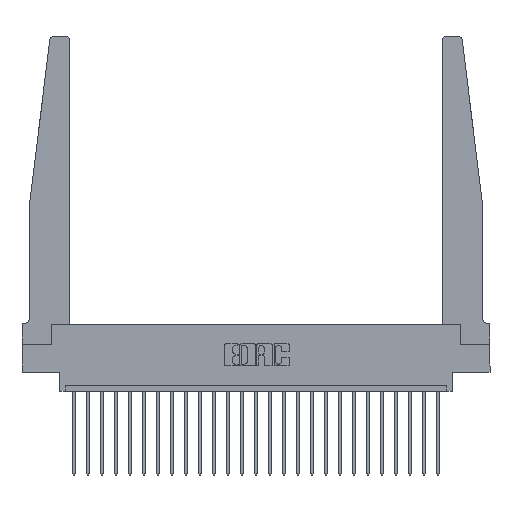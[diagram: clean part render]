
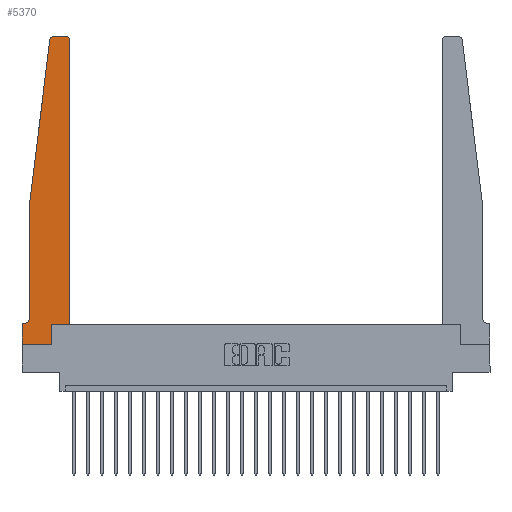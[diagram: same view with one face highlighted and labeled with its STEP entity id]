
A CAD part, top view. The second image highlights one B-rep face of the part: STEP entity #5370.
In plain terms, the highlighted planar face has unit normal (0, 0, 1).
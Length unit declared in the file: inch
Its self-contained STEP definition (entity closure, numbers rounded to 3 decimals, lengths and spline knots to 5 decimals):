
#117 = EDGE_CURVE ( 'NONE', #17860, #14501, #14107, .T. ) ;
#538 = AXIS2_PLACEMENT_3D ( 'NONE', #19461, #14098, #1258 ) ;
#866 = CARTESIAN_POINT ( 'NONE',  ( 0.2605, 0., 0.37 ) ) ;
#1106 = VECTOR ( 'NONE', #4166, 39.37008 ) ;
#1123 = AXIS2_PLACEMENT_3D ( 'NONE', #10240, #10121, #8539 ) ;
#1258 = DIRECTION ( 'NONE',  ( 1., 0., 0. ) ) ;
#1379 = LINE ( 'NONE', #3693, #8368 ) ;
#1719 = CARTESIAN_POINT ( 'NONE',  ( 0., 0., 0.37 ) ) ;
#1880 = DIRECTION ( 'NONE',  ( 0., -1., 0. ) ) ;
#2610 = AXIS2_PLACEMENT_3D ( 'NONE', #13064, #20389, #16616 ) ;
#2617 = DIRECTION ( 'NONE',  ( 0., 1., 0. ) ) ;
#2806 = ORIENTED_EDGE ( 'NONE', *, *, #21294, .T. ) ;
#2955 = VECTOR ( 'NONE', #18451, 39.37008 ) ;
#3635 = VERTEX_POINT ( 'NONE', #22737 ) ;
#3693 = CARTESIAN_POINT ( 'NONE',  ( 0.065, 1.25, 0.37 ) ) ;
#3705 = ORIENTED_EDGE ( 'NONE', *, *, #21782, .T. ) ;
#4132 = CARTESIAN_POINT ( 'NONE',  ( 0., 0., 0.37 ) ) ;
#4146 = ORIENTED_EDGE ( 'NONE', *, *, #23556, .T. ) ;
#4166 = DIRECTION ( 'NONE',  ( 0., 1., 0. ) ) ;
#4489 = ORIENTED_EDGE ( 'NONE', *, *, #9427, .T. ) ;
#4519 = EDGE_CURVE ( 'NONE', #5183, #11745, #11567, .T. ) ;
#4867 = VECTOR ( 'NONE', #2617, 39.37008 ) ;
#4907 = CARTESIAN_POINT ( 'NONE',  ( 0.065, 1.25, 0.37 ) ) ;
#4926 = VECTOR ( 'NONE', #9857, 39.37008 ) ;
#4960 = LINE ( 'NONE', #6920, #7744 ) ;
#5116 = CARTESIAN_POINT ( 'NONE',  ( 0.065, 0.2375, 0.37 ) ) ;
#5183 = VERTEX_POINT ( 'NONE', #22739 ) ;
#5370 = ADVANCED_FACE ( 'NONE', ( #12104 ), #11985, .T. ) ;
#5738 = EDGE_CURVE ( 'NONE', #11604, #5183, #4960, .T. ) ;
#5764 = VECTOR ( 'NONE', #16285, 39.37008 ) ;
#6403 = CARTESIAN_POINT ( 'NONE',  ( 0.425, 0.18, 0.37 ) ) ;
#6478 = DIRECTION ( 'NONE',  ( 1., 0., 0. ) ) ;
#6920 = CARTESIAN_POINT ( 'NONE',  ( 0.065, 0.1875, 0.37 ) ) ;
#7546 = DIRECTION ( 'NONE',  ( 0., -1., 0. ) ) ;
#7744 = VECTOR ( 'NONE', #14486, 39.37008 ) ;
#7966 = CIRCLE ( 'NONE', #538, 0.03 ) ;
#8003 = LINE ( 'NONE', #15459, #10424 ) ;
#8266 = LINE ( 'NONE', #6403, #4926 ) ;
#8336 = LINE ( 'NONE', #1719, #2955 ) ;
#8368 = VECTOR ( 'NONE', #1880, 39.37008 ) ;
#8539 = DIRECTION ( 'NONE',  ( -1., 0., 0. ) ) ;
#9427 = EDGE_CURVE ( 'NONE', #14501, #19465, #15128, .T. ) ;
#9755 = CARTESIAN_POINT ( 'NONE',  ( 0., 0., 0.37 ) ) ;
#9857 = DIRECTION ( 'NONE',  ( 1., 0., 0. ) ) ;
#10121 = DIRECTION ( 'NONE',  ( 0., 0., -1. ) ) ;
#10161 = CARTESIAN_POINT ( 'NONE',  ( 0., 0.1875, 0.37 ) ) ;
#10240 = CARTESIAN_POINT ( 'NONE',  ( 0.015, 0.2375, 0.37 ) ) ;
#10290 = CARTESIAN_POINT ( 'NONE',  ( 0.425, 2.72, 0.37 ) ) ;
#10424 = VECTOR ( 'NONE', #10816, 39.37008 ) ;
#10498 = ORIENTED_EDGE ( 'NONE', *, *, #5738, .T. ) ;
#10816 = DIRECTION ( 'NONE',  ( -1., 0., 0. ) ) ;
#10876 = AXIS2_PLACEMENT_3D ( 'NONE', #10161, #23206, #6478 ) ;
#11039 = EDGE_CURVE ( 'NONE', #15997, #17860, #8266, .T. ) ;
#11567 = LINE ( 'NONE', #9755, #17832 ) ;
#11604 = VERTEX_POINT ( 'NONE', #12500 ) ;
#11745 = VERTEX_POINT ( 'NONE', #4132 ) ;
#11985 = PLANE ( 'NONE',  #10876 ) ;
#12104 = FACE_OUTER_BOUND ( 'NONE', #21296, .T. ) ;
#12475 = VERTEX_POINT ( 'NONE', #22285 ) ;
#12500 = CARTESIAN_POINT ( 'NONE',  ( 0.015, 0.1875, 0.37 ) ) ;
#12958 = ORIENTED_EDGE ( 'NONE', *, *, #117, .T. ) ;
#13060 = EDGE_CURVE ( 'NONE', #12475, #3635, #7966, .T. ) ;
#13064 = CARTESIAN_POINT ( 'NONE',  ( 0.395, 2.72, 0.37 ) ) ;
#13222 = EDGE_CURVE ( 'NONE', #18788, #18901, #1379, .T. ) ;
#13319 = ORIENTED_EDGE ( 'NONE', *, *, #13060, .T. ) ;
#13683 = CARTESIAN_POINT ( 'NONE',  ( 0.065, 1.25, 0.37 ) ) ;
#14098 = DIRECTION ( 'NONE',  ( 0., 0., 1. ) ) ;
#14107 = LINE ( 'NONE', #17640, #4867 ) ;
#14486 = DIRECTION ( 'NONE',  ( -1., 0., 0. ) ) ;
#14501 = VERTEX_POINT ( 'NONE', #10290 ) ;
#14985 = CARTESIAN_POINT ( 'NONE',  ( 0.395, 2.75, 0.37 ) ) ;
#15128 = CIRCLE ( 'NONE', #2610, 0.03 ) ;
#15459 = CARTESIAN_POINT ( 'NONE',  ( 0.25, 2.75, 0.37 ) ) ;
#15997 = VERTEX_POINT ( 'NONE', #16132 ) ;
#16132 = CARTESIAN_POINT ( 'NONE',  ( 0.2605, 0.18, 0.37 ) ) ;
#16285 = DIRECTION ( 'NONE',  ( -0.122, -0.992, 0. ) ) ;
#16616 = DIRECTION ( 'NONE',  ( 1., 0., 0. ) ) ;
#17139 = ORIENTED_EDGE ( 'NONE', *, *, #24050, .T. ) ;
#17618 = ORIENTED_EDGE ( 'NONE', *, *, #18381, .T. ) ;
#17640 = CARTESIAN_POINT ( 'NONE',  ( 0.425, 0.18, 0.37 ) ) ;
#17832 = VECTOR ( 'NONE', #7546, 39.37008 ) ;
#17860 = VERTEX_POINT ( 'NONE', #23492 ) ;
#18378 = VERTEX_POINT ( 'NONE', #866 ) ;
#18381 = EDGE_CURVE ( 'NONE', #11745, #18378, #8336, .T. ) ;
#18390 = ORIENTED_EDGE ( 'NONE', *, *, #4519, .T. ) ;
#18451 = DIRECTION ( 'NONE',  ( 1., 0., 0. ) ) ;
#18788 = VERTEX_POINT ( 'NONE', #13683 ) ;
#18901 = VERTEX_POINT ( 'NONE', #5116 ) ;
#19461 = CARTESIAN_POINT ( 'NONE',  ( 0.27653, 2.72, 0.37 ) ) ;
#19463 = CIRCLE ( 'NONE', #1123, 0.05 ) ;
#19465 = VERTEX_POINT ( 'NONE', #14985 ) ;
#19680 = LINE ( 'NONE', #4907, #5764 ) ;
#20389 = DIRECTION ( 'NONE',  ( 0., 0., 1. ) ) ;
#20835 = ORIENTED_EDGE ( 'NONE', *, *, #13222, .T. ) ;
#20903 = CARTESIAN_POINT ( 'NONE',  ( 0.2605, 0.18, 0.37 ) ) ;
#21294 = EDGE_CURVE ( 'NONE', #19465, #12475, #8003, .T. ) ;
#21296 = EDGE_LOOP ( 'NONE', ( #2806, #13319, #3705, #20835, #17139, #10498, #18390, #17618, #4146, #23177, #12958, #4489 ) ) ;
#21782 = EDGE_CURVE ( 'NONE', #3635, #18788, #19680, .T. ) ;
#22285 = CARTESIAN_POINT ( 'NONE',  ( 0.27653, 2.75, 0.37 ) ) ;
#22733 = LINE ( 'NONE', #20903, #1106 ) ;
#22737 = CARTESIAN_POINT ( 'NONE',  ( 0.24675, 2.72367, 0.37 ) ) ;
#22739 = CARTESIAN_POINT ( 'NONE',  ( 0., 0.1875, 0.37 ) ) ;
#23177 = ORIENTED_EDGE ( 'NONE', *, *, #11039, .T. ) ;
#23206 = DIRECTION ( 'NONE',  ( 0., 0., 1. ) ) ;
#23492 = CARTESIAN_POINT ( 'NONE',  ( 0.425, 0.18, 0.37 ) ) ;
#23556 = EDGE_CURVE ( 'NONE', #18378, #15997, #22733, .T. ) ;
#24050 = EDGE_CURVE ( 'NONE', #18901, #11604, #19463, .T. ) ;
